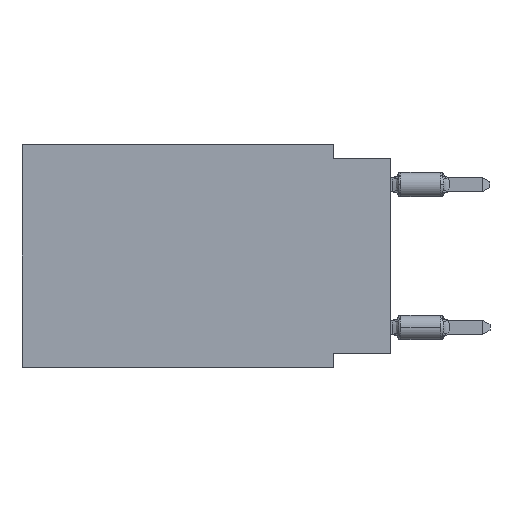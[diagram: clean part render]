
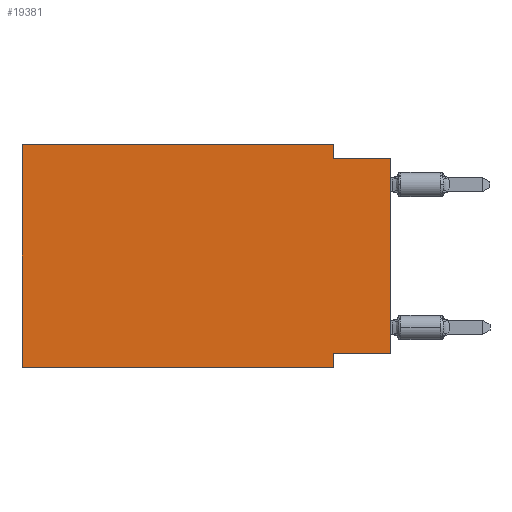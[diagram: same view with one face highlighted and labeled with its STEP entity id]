
A CAD part, left-side view. The second image highlights one B-rep face of the part: STEP entity #19381.
In plain terms, the highlighted planar face has unit normal (-1, 0, 0).
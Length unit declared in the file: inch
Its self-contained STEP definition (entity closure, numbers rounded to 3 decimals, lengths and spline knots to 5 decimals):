
#520 = EDGE_CURVE ( 'NONE', #921, #3625, #23921, .T. ) ;
#530 = CARTESIAN_POINT ( 'NONE',  ( 0., 0.645, 0. ) ) ;
#921 = VERTEX_POINT ( 'NONE', #16744 ) ;
#1280 = CARTESIAN_POINT ( 'NONE',  ( 0., 0.645, -0.39 ) ) ;
#1354 = ORIENTED_EDGE ( 'NONE', *, *, #22100, .F. ) ;
#2173 = DIRECTION ( 'NONE',  ( 0., 0., 1. ) ) ;
#2538 = DIRECTION ( 'NONE',  ( 0., 0., -1. ) ) ;
#2653 = CARTESIAN_POINT ( 'NONE',  ( 0., 0.1, 0. ) ) ;
#3143 = PLANE ( 'NONE',  #16068 ) ;
#3625 = VERTEX_POINT ( 'NONE', #10214 ) ;
#3884 = EDGE_CURVE ( 'NONE', #14416, #9303, #32681, .T. ) ;
#4383 = CARTESIAN_POINT ( 'NONE',  ( 0., 0., -0.365 ) ) ;
#5591 = CARTESIAN_POINT ( 'NONE',  ( 0., 0., 0. ) ) ;
#6984 = VECTOR ( 'NONE', #27016, 39.37008 ) ;
#7965 = VECTOR ( 'NONE', #15363, 39.37008 ) ;
#8505 = DIRECTION ( 'NONE',  ( 0., 0., -1. ) ) ;
#8986 = VECTOR ( 'NONE', #2173, 39.37008 ) ;
#9303 = VERTEX_POINT ( 'NONE', #33885 ) ;
#10113 = VECTOR ( 'NONE', #16755, 39.37008 ) ;
#10214 = CARTESIAN_POINT ( 'NONE',  ( 0., 0., -0.025 ) ) ;
#10274 = ORIENTED_EDGE ( 'NONE', *, *, #18898, .F. ) ;
#10663 = LINE ( 'NONE', #33841, #23186 ) ;
#11090 = DIRECTION ( 'NONE',  ( 1., 0., 0. ) ) ;
#11575 = EDGE_CURVE ( 'NONE', #33484, #12786, #16316, .T. ) ;
#12031 = CARTESIAN_POINT ( 'NONE',  ( 0., 0.1, -0.365 ) ) ;
#12779 = LINE ( 'NONE', #18135, #7965 ) ;
#12786 = VERTEX_POINT ( 'NONE', #12031 ) ;
#13257 = ORIENTED_EDGE ( 'NONE', *, *, #11575, .F. ) ;
#13576 = VECTOR ( 'NONE', #22614, 39.37008 ) ;
#14001 = CARTESIAN_POINT ( 'NONE',  ( 0., 0.645, 0. ) ) ;
#14416 = VERTEX_POINT ( 'NONE', #1280 ) ;
#14438 = CARTESIAN_POINT ( 'NONE',  ( 0., 0.645, -0.39 ) ) ;
#15363 = DIRECTION ( 'NONE',  ( 0., 0., -1. ) ) ;
#15873 = VERTEX_POINT ( 'NONE', #2653 ) ;
#16068 = AXIS2_PLACEMENT_3D ( 'NONE', #530, #11090, #8505 ) ;
#16316 = LINE ( 'NONE', #29644, #6984 ) ;
#16328 = EDGE_CURVE ( 'NONE', #14416, #32097, #17026, .T. ) ;
#16744 = CARTESIAN_POINT ( 'NONE',  ( 0., 0.1, -0.025 ) ) ;
#16755 = DIRECTION ( 'NONE',  ( 0., -1., 0. ) ) ;
#17026 = LINE ( 'NONE', #14438, #32570 ) ;
#18135 = CARTESIAN_POINT ( 'NONE',  ( 0., 0.1, 0. ) ) ;
#18585 = CARTESIAN_POINT ( 'NONE',  ( 0., 0., -0.025 ) ) ;
#18898 = EDGE_CURVE ( 'NONE', #12786, #32097, #10663, .T. ) ;
#19381 = ADVANCED_FACE ( 'NONE', ( #29421 ), #3143, .F. ) ;
#19513 = ORIENTED_EDGE ( 'NONE', *, *, #16328, .T. ) ;
#19863 = CARTESIAN_POINT ( 'NONE',  ( 0., 0.645, 0. ) ) ;
#21618 = EDGE_CURVE ( 'NONE', #33484, #3625, #32056, .T. ) ;
#22100 = EDGE_CURVE ( 'NONE', #9303, #15873, #22447, .T. ) ;
#22447 = LINE ( 'NONE', #19863, #10113 ) ;
#22614 = DIRECTION ( 'NONE',  ( 0., 0., 1. ) ) ;
#23186 = VECTOR ( 'NONE', #2538, 39.37008 ) ;
#23921 = LINE ( 'NONE', #18585, #30085 ) ;
#24422 = DIRECTION ( 'NONE',  ( 0., -1., 0. ) ) ;
#24652 = EDGE_LOOP ( 'NONE', ( #34171, #26343, #31610, #1354, #28248, #19513, #10274, #13257 ) ) ;
#26343 = ORIENTED_EDGE ( 'NONE', *, *, #520, .F. ) ;
#27016 = DIRECTION ( 'NONE',  ( 0., 1., 0. ) ) ;
#27301 = CARTESIAN_POINT ( 'NONE',  ( 0., 0.1, -0.39 ) ) ;
#27310 = EDGE_CURVE ( 'NONE', #15873, #921, #12779, .T. ) ;
#28248 = ORIENTED_EDGE ( 'NONE', *, *, #3884, .F. ) ;
#29421 = FACE_OUTER_BOUND ( 'NONE', #24652, .T. ) ;
#29644 = CARTESIAN_POINT ( 'NONE',  ( 0., 0., -0.365 ) ) ;
#30006 = DIRECTION ( 'NONE',  ( 0., -1., 0. ) ) ;
#30085 = VECTOR ( 'NONE', #24422, 39.37008 ) ;
#31610 = ORIENTED_EDGE ( 'NONE', *, *, #27310, .F. ) ;
#32056 = LINE ( 'NONE', #5591, #8986 ) ;
#32097 = VERTEX_POINT ( 'NONE', #27301 ) ;
#32570 = VECTOR ( 'NONE', #30006, 39.37008 ) ;
#32681 = LINE ( 'NONE', #14001, #13576 ) ;
#33484 = VERTEX_POINT ( 'NONE', #4383 ) ;
#33841 = CARTESIAN_POINT ( 'NONE',  ( 0., 0.1, -0.39 ) ) ;
#33885 = CARTESIAN_POINT ( 'NONE',  ( 0., 0.645, 0. ) ) ;
#34171 = ORIENTED_EDGE ( 'NONE', *, *, #21618, .T. ) ;
